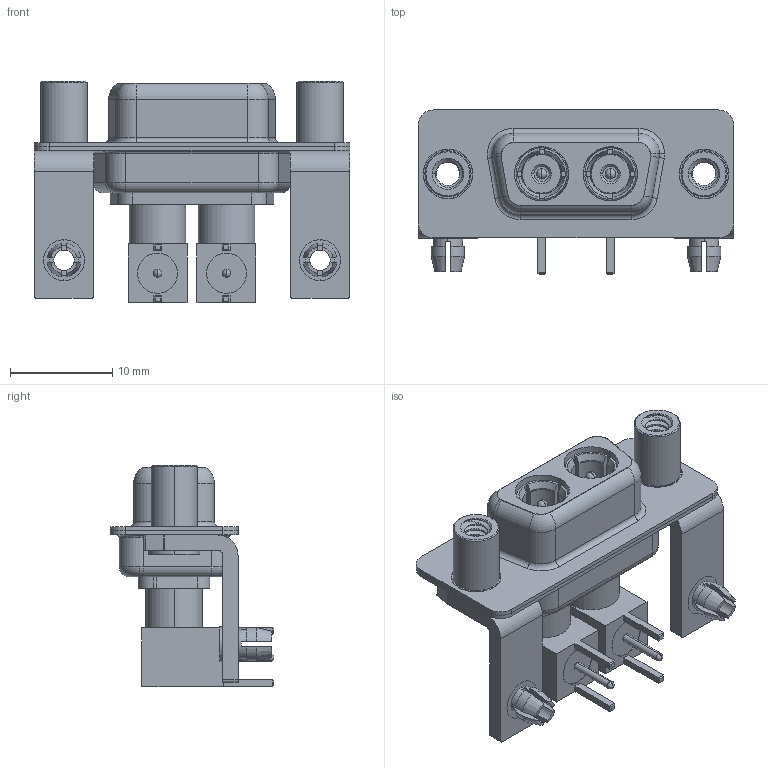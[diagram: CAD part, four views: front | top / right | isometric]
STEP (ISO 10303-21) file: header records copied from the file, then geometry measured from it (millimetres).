
FILE_DESCRIPTION (( 'STEP AP203' ), '1' );
FILE_NAME ('630-2W2-640-7N5.STEP', '2022-05-26T19:47:58', ( '' ), ( '' ), 'SwSTEP 2.0', 'SolidWorks 2020', '' );
FILE_SCHEMA (( 'CONFIG_CONTROL_DESIGN' ));
Length unit declared in the file: millimetre
Products named in the file (15): 630Combo Threaded Standoff_5; Locking Collar; Co-Ax Plug Assy_RA; RA Back Shell; 630Combo Shell Rear_09 Contacts; 630Combo Board Lock; 630Combo Housing_2W2; 630Combo Stabilizer Bracket; Insulator Pin_Straight PC Tail; Pin_RA; Insulator RA Pin; 630Combo Shell Front_09 Contacts; 630-2W2-640-7N5; Co-Ax Plug_RA PC Tail
Assembly tree (23 placements, depth 3):
  630-2W2-640-7N5
    630Combo Housing_2W2
    630Combo Shell Front_09 Contacts
    630Combo Shell Rear_09 Contacts
    630Combo Stabilizer Bracket  x2
    630Combo Board Lock  x2
    630Combo Threaded Standoff_5  x2
    Co-Ax Plug Assy_RA
      Co-Ax Plug_RA PC Tail
      Insulator Pin_Straight PC Tail
      Pin_RA
      Locking Collar
      RA Back Shell
      Insulator RA Pin
    Co-Ax Plug Assy_RA
      Co-Ax Plug_RA PC Tail
      Insulator Pin_Straight PC Tail
      Pin_RA
      Locking Collar
      RA Back Shell
      Insulator RA Pin
Bounding box: 30.8 x 16 x 21.61 mm (x, y, z)
Volume: 2570.8 mm3; surface area: 6761.5 mm2
Topology: 21 solids, 21 shells, 795 faces, 1971 edges, 1247 vertices
Faces by surface type: cylinder 359, plane 271, cone 80, torus 69, bspline 8, sphere 8
Entity records: 19007 total; most frequent: CARTESIAN_POINT 4924, DIRECTION 2717, ORIENTED_EDGE 2494, EDGE_CURVE 1247, AXIS2_PLACEMENT_3D 1080, VERTEX_POINT 791, EDGE_LOOP 570, VECTOR 557
